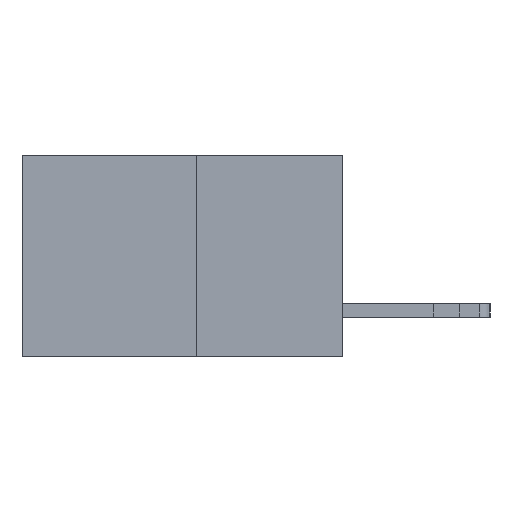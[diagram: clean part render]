
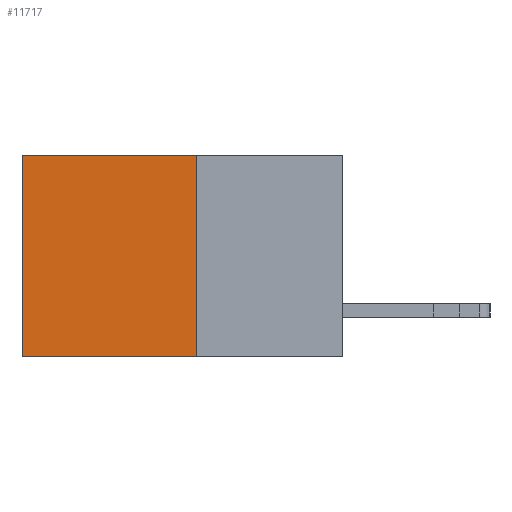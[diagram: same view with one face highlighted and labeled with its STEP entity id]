
A CAD part, left-side view. The second image highlights one B-rep face of the part: STEP entity #11717.
In plain terms, the highlighted planar face has unit normal (-1, 0, 0).
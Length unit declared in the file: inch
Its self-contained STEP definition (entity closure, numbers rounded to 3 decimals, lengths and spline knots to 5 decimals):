
#955 = CARTESIAN_POINT ( 'NONE',  ( 0.277, 0.27, -0.37 ) ) ;
#969 = EDGE_CURVE ( 'NONE', #5113, #12251, #10037, .T. ) ;
#1319 = EDGE_CURVE ( 'NONE', #6293, #12251, #1407, .T. ) ;
#1407 = LINE ( 'NONE', #6452, #7338 ) ;
#1994 = ORIENTED_EDGE ( 'NONE', *, *, #1319, .T. ) ;
#2017 = VECTOR ( 'NONE', #14277, 39.37008 ) ;
#2149 = DIRECTION ( 'NONE',  ( 0., 0., -1. ) ) ;
#2403 = LINE ( 'NONE', #7522, #2017 ) ;
#2572 = CARTESIAN_POINT ( 'NONE',  ( 0.277, 0.27, -0.37 ) ) ;
#2589 = DIRECTION ( 'NONE',  ( 0., 1., 0. ) ) ;
#2746 = VECTOR ( 'NONE', #2589, 39.37008 ) ;
#2973 = CARTESIAN_POINT ( 'NONE',  ( 0.277, 0.27, -0.37 ) ) ;
#2993 = DIRECTION ( 'NONE',  ( 0., 0., -1. ) ) ;
#4686 = VERTEX_POINT ( 'NONE', #14406 ) ;
#5113 = VERTEX_POINT ( 'NONE', #13402 ) ;
#5203 = ORIENTED_EDGE ( 'NONE', *, *, #969, .F. ) ;
#5446 = CARTESIAN_POINT ( 'NONE',  ( 0.277, 0.59, -0.37 ) ) ;
#5709 = PLANE ( 'NONE',  #14752 ) ;
#5849 = EDGE_LOOP ( 'NONE', ( #1994, #5203, #10951, #7935 ) ) ;
#6121 = LINE ( 'NONE', #2973, #14769 ) ;
#6293 = VERTEX_POINT ( 'NONE', #6748 ) ;
#6452 = CARTESIAN_POINT ( 'NONE',  ( 0.277, 0.59, -0.37 ) ) ;
#6620 = DIRECTION ( 'NONE',  ( 0., 0., -1. ) ) ;
#6748 = CARTESIAN_POINT ( 'NONE',  ( 0.277, 0.59, 0. ) ) ;
#7202 = EDGE_CURVE ( 'NONE', #4686, #5113, #6121, .T. ) ;
#7338 = VECTOR ( 'NONE', #6620, 39.37008 ) ;
#7522 = CARTESIAN_POINT ( 'NONE',  ( 0.277, 0.27, 0. ) ) ;
#7935 = ORIENTED_EDGE ( 'NONE', *, *, #9670, .T. ) ;
#8939 = FACE_OUTER_BOUND ( 'NONE', #5849, .T. ) ;
#9180 = DIRECTION ( 'NONE',  ( 1., 0., 0. ) ) ;
#9670 = EDGE_CURVE ( 'NONE', #4686, #6293, #2403, .T. ) ;
#10037 = LINE ( 'NONE', #2572, #2746 ) ;
#10951 = ORIENTED_EDGE ( 'NONE', *, *, #7202, .F. ) ;
#11717 = ADVANCED_FACE ( 'NONE', ( #8939 ), #5709, .F. ) ;
#12251 = VERTEX_POINT ( 'NONE', #5446 ) ;
#13402 = CARTESIAN_POINT ( 'NONE',  ( 0.277, 0.27, -0.37 ) ) ;
#14277 = DIRECTION ( 'NONE',  ( 0., 1., 0. ) ) ;
#14406 = CARTESIAN_POINT ( 'NONE',  ( 0.277, 0.27, 0. ) ) ;
#14752 = AXIS2_PLACEMENT_3D ( 'NONE', #955, #9180, #2149 ) ;
#14769 = VECTOR ( 'NONE', #2993, 39.37008 ) ;
